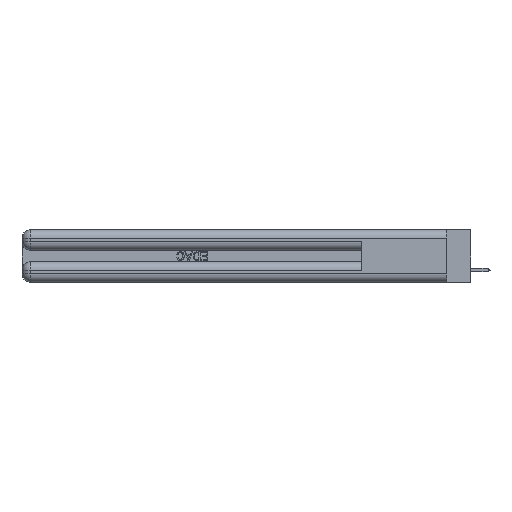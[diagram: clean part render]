
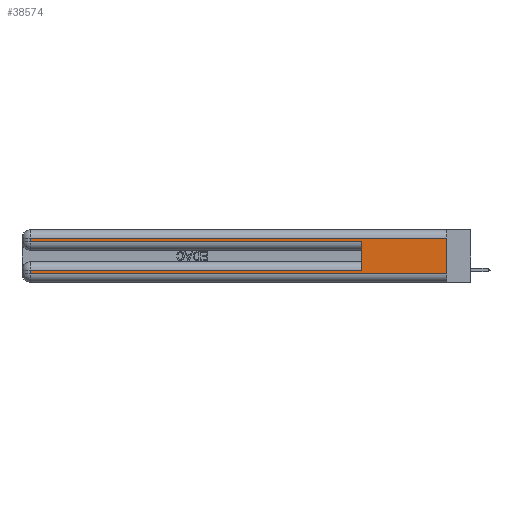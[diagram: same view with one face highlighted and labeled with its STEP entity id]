
A CAD part, left-side view. The second image highlights one B-rep face of the part: STEP entity #38574.
In plain terms, the highlighted planar face has unit normal (-1, 0, 0).
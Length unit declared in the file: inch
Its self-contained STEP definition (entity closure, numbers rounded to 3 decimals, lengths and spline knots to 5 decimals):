
#4280 = EDGE_CURVE ( 'NONE', #42752, #46745, #16166, .T. ) ;
#4974 = ORIENTED_EDGE ( 'NONE', *, *, #29003, .T. ) ;
#5300 = EDGE_CURVE ( 'NONE', #37110, #34932, #5953, .T. ) ;
#5728 = EDGE_CURVE ( 'NONE', #24682, #50859, #13993, .T. ) ;
#5953 = LINE ( 'NONE', #19882, #19208 ) ;
#8117 = VECTOR ( 'NONE', #12009, 39.37008 ) ;
#8223 = VECTOR ( 'NONE', #37230, 39.37008 ) ;
#8675 = DIRECTION ( 'NONE',  ( 0., -1., 0. ) ) ;
#10095 = ORIENTED_EDGE ( 'NONE', *, *, #5728, .T. ) ;
#11234 = CARTESIAN_POINT ( 'NONE',  ( 0., 0., 0.085 ) ) ;
#12009 = DIRECTION ( 'NONE',  ( 0., 1., 0. ) ) ;
#13993 = LINE ( 'NONE', #54304, #23203 ) ;
#14110 = ORIENTED_EDGE ( 'NONE', *, *, #4280, .T. ) ;
#14479 = AXIS2_PLACEMENT_3D ( 'NONE', #44951, #17048, #46258 ) ;
#14962 = VERTEX_POINT ( 'NONE', #27762 ) ;
#16166 = LINE ( 'NONE', #54188, #8223 ) ;
#17048 = DIRECTION ( 'NONE',  ( 1., 0., 0. ) ) ;
#18481 = CARTESIAN_POINT ( 'NONE',  ( 0., 2.94, 0.285 ) ) ;
#18936 = DIRECTION ( 'NONE',  ( 0., 0., 1. ) ) ;
#19208 = VECTOR ( 'NONE', #19679, 39.37008 ) ;
#19679 = DIRECTION ( 'NONE',  ( 0., 0., -1. ) ) ;
#19882 = CARTESIAN_POINT ( 'NONE',  ( 0., 0., 0.37 ) ) ;
#20357 = EDGE_CURVE ( 'NONE', #14962, #46745, #44163, .T. ) ;
#20485 = EDGE_CURVE ( 'NONE', #37110, #54338, #21686, .T. ) ;
#21640 = CARTESIAN_POINT ( 'NONE',  ( 0., 0., 0.31 ) ) ;
#21686 = LINE ( 'NONE', #21640, #22285 ) ;
#22100 = LINE ( 'NONE', #28991, #32875 ) ;
#22285 = VECTOR ( 'NONE', #38873, 39.37008 ) ;
#23203 = VECTOR ( 'NONE', #28985, 39.37008 ) ;
#23763 = ORIENTED_EDGE ( 'NONE', *, *, #20357, .F. ) ;
#24682 = VERTEX_POINT ( 'NONE', #52058 ) ;
#25600 = EDGE_LOOP ( 'NONE', ( #43042, #28513, #49012, #14110, #23763, #4974, #10095, #36049 ) ) ;
#26091 = FACE_OUTER_BOUND ( 'NONE', #25600, .T. ) ;
#26540 = EDGE_CURVE ( 'NONE', #54338, #42752, #22100, .T. ) ;
#27663 = LINE ( 'NONE', #35812, #45582 ) ;
#27762 = CARTESIAN_POINT ( 'NONE',  ( 0., 0.6, 0.085 ) ) ;
#28513 = ORIENTED_EDGE ( 'NONE', *, *, #20485, .T. ) ;
#28612 = DIRECTION ( 'NONE',  ( 0., 0., -1. ) ) ;
#28985 = DIRECTION ( 'NONE',  ( 0., 0., -1. ) ) ;
#28991 = CARTESIAN_POINT ( 'NONE',  ( 0., 2.94, 0.37 ) ) ;
#29003 = EDGE_CURVE ( 'NONE', #14962, #24682, #53703, .T. ) ;
#32875 = VECTOR ( 'NONE', #28612, 39.37008 ) ;
#34932 = VERTEX_POINT ( 'NONE', #53836 ) ;
#35217 = CARTESIAN_POINT ( 'NONE',  ( 0., 2.94, 0.06 ) ) ;
#35812 = CARTESIAN_POINT ( 'NONE',  ( 0., 0., 0.06 ) ) ;
#36049 = ORIENTED_EDGE ( 'NONE', *, *, #40122, .T. ) ;
#37110 = VERTEX_POINT ( 'NONE', #48158 ) ;
#37121 = CARTESIAN_POINT ( 'NONE',  ( 0., 2.94, 0.31 ) ) ;
#37230 = DIRECTION ( 'NONE',  ( 0., -1., 0. ) ) ;
#38574 = ADVANCED_FACE ( 'NONE', ( #26091 ), #45350, .F. ) ;
#38873 = DIRECTION ( 'NONE',  ( 0., 1., 0. ) ) ;
#40122 = EDGE_CURVE ( 'NONE', #50859, #34932, #27663, .T. ) ;
#42752 = VERTEX_POINT ( 'NONE', #18481 ) ;
#43042 = ORIENTED_EDGE ( 'NONE', *, *, #5300, .F. ) ;
#44163 = LINE ( 'NONE', #52234, #53513 ) ;
#44951 = CARTESIAN_POINT ( 'NONE',  ( 0., 0., 0.37 ) ) ;
#45350 = PLANE ( 'NONE',  #14479 ) ;
#45582 = VECTOR ( 'NONE', #8675, 39.37008 ) ;
#46258 = DIRECTION ( 'NONE',  ( 0., 0., -1. ) ) ;
#46745 = VERTEX_POINT ( 'NONE', #51428 ) ;
#48158 = CARTESIAN_POINT ( 'NONE',  ( 0., 0., 0.31 ) ) ;
#49012 = ORIENTED_EDGE ( 'NONE', *, *, #26540, .T. ) ;
#50859 = VERTEX_POINT ( 'NONE', #35217 ) ;
#51428 = CARTESIAN_POINT ( 'NONE',  ( 0., 0.6, 0.285 ) ) ;
#52058 = CARTESIAN_POINT ( 'NONE',  ( 0., 2.94, 0.085 ) ) ;
#52234 = CARTESIAN_POINT ( 'NONE',  ( 0., 0.6, 0.145 ) ) ;
#53513 = VECTOR ( 'NONE', #18936, 39.37008 ) ;
#53703 = LINE ( 'NONE', #11234, #8117 ) ;
#53836 = CARTESIAN_POINT ( 'NONE',  ( 0., 0., 0.06 ) ) ;
#54188 = CARTESIAN_POINT ( 'NONE',  ( 0., 0., 0.285 ) ) ;
#54304 = CARTESIAN_POINT ( 'NONE',  ( 0., 2.94, 0.37 ) ) ;
#54338 = VERTEX_POINT ( 'NONE', #37121 ) ;
